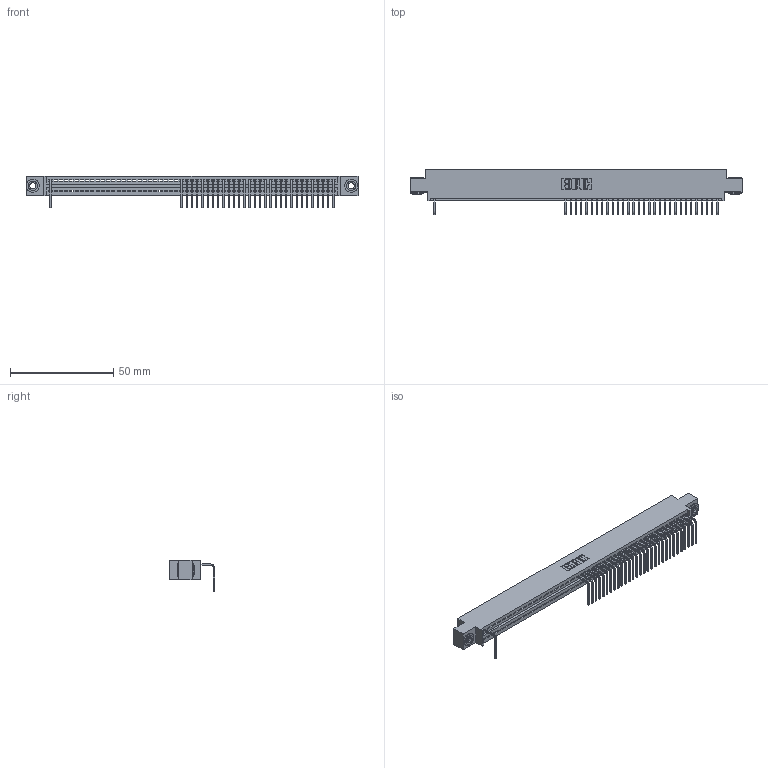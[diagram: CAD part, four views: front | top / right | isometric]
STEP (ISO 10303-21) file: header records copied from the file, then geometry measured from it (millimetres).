
FILE_DESCRIPTION (( 'STEP AP203' ), '1' );
FILE_NAME ('345-055-558-603.STEP', '2018-09-24T05:39:29', ( '' ), ( '' ), 'SwSTEP 2.0', 'SolidWorks 2016', '' );
FILE_SCHEMA (( 'CONFIG_CONTROL_DESIGN' ));
Length unit declared in the file: inch
Products named in the file (4): 345 Part_0.170 Offset - 0.156 Dia-TH; 345-292-001_558 Tail - 2; 345-250-002_345-250-002-102; 345-055-558-603
Assembly tree (34 placements, depth 2):
  345-055-558-603
    345 Part_0.170 Offset - 0.156 Dia-TH
    345-292-001_558 Tail - 2  x31
    345-250-002_345-250-002-102  x2
Bounding box: 160.91 x 21.83 x 15.37 mm (x, y, z)
Volume: 15124.3 mm3; surface area: 19764 mm2
Topology: 34 solids, 34 shells, 2412 faces, 7367 edges, 4866 vertices
Faces by surface type: plane 1732, cylinder 672, cone 8
Entity records: 39742 total; most frequent: ORIENTED_EDGE 6978, CARTESIAN_POINT 6972, DIRECTION 6073, EDGE_CURVE 3489, VECTOR 3113, LINE 3113, VERTEX_POINT 2322, AXIS2_PLACEMENT_3D 1480
